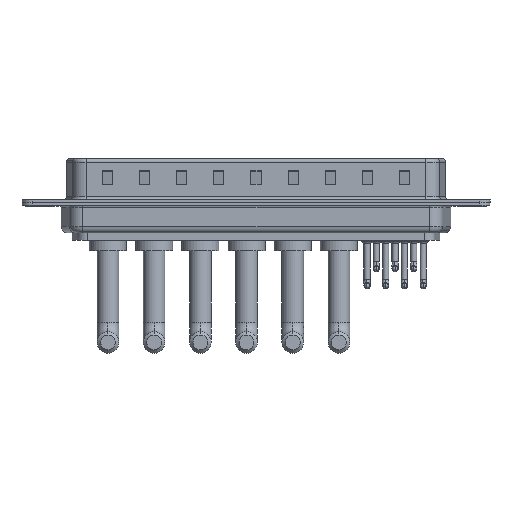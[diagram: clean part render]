
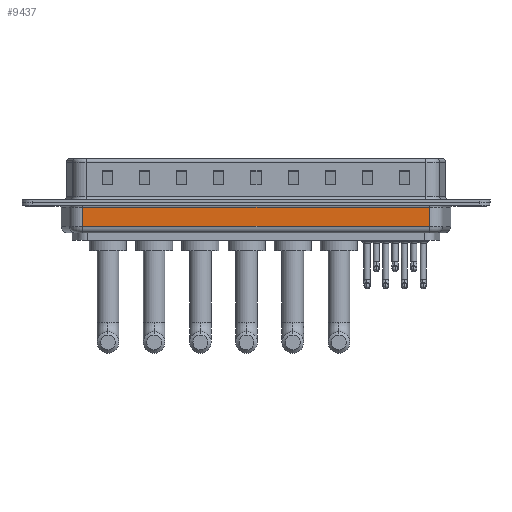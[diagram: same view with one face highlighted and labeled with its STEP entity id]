
A CAD part, front view. The second image highlights one B-rep face of the part: STEP entity #9437.
In plain terms, the highlighted planar face has unit normal (0, -1, 0).
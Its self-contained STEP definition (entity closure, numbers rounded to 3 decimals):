
#38 = VECTOR ( 'NONE', #15223, 1000. ) ;
#394 = CARTESIAN_POINT ( 'NONE',  ( 6.031, -5.35, -4.5 ) ) ;
#1238 = CARTESIAN_POINT ( 'NONE',  ( 57.469, -5.35, -3.5 ) ) ;
#1343 = VERTEX_POINT ( 'NONE', #16554 ) ;
#4052 = DIRECTION ( 'NONE',  ( -1., 0., 0. ) ) ;
#4387 = DIRECTION ( 'NONE',  ( 0., 0., 1. ) ) ;
#5097 = CARTESIAN_POINT ( 'NONE',  ( 6.031, -5.35, -0.65 ) ) ;
#5943 = VERTEX_POINT ( 'NONE', #10109 ) ;
#6286 = ORIENTED_EDGE ( 'NONE', *, *, #9462, .F. ) ;
#7620 = VERTEX_POINT ( 'NONE', #1238 ) ;
#8162 = ORIENTED_EDGE ( 'NONE', *, *, #16413, .T. ) ;
#8227 = CARTESIAN_POINT ( 'NONE',  ( 6.031, -5.35, -3.5 ) ) ;
#9286 = VECTOR ( 'NONE', #19094, 1000. ) ;
#9437 = ADVANCED_FACE ( 'NONE', ( #21397 ), #14633, .F. ) ;
#9462 = EDGE_CURVE ( 'NONE', #17589, #1343, #14866, .T. ) ;
#9883 = EDGE_CURVE ( 'NONE', #17589, #7620, #13262, .T. ) ;
#10109 = CARTESIAN_POINT ( 'NONE',  ( 57.469, -5.35, -0.65 ) ) ;
#10959 = CARTESIAN_POINT ( 'NONE',  ( 6.031, -5.35, -4.5 ) ) ;
#11719 = EDGE_CURVE ( 'NONE', #5943, #1343, #13826, .T. ) ;
#12854 = AXIS2_PLACEMENT_3D ( 'NONE', #10959, #17969, #4052 ) ;
#13262 = LINE ( 'NONE', #8227, #38 ) ;
#13292 = ORIENTED_EDGE ( 'NONE', *, *, #9883, .T. ) ;
#13826 = LINE ( 'NONE', #5097, #9286 ) ;
#14226 = EDGE_LOOP ( 'NONE', ( #6286, #13292, #8162, #15692 ) ) ;
#14633 = PLANE ( 'NONE',  #12854 ) ;
#14866 = LINE ( 'NONE', #394, #15432 ) ;
#15223 = DIRECTION ( 'NONE',  ( 1., 0., 0. ) ) ;
#15356 = DIRECTION ( 'NONE',  ( 0., 0., 1. ) ) ;
#15432 = VECTOR ( 'NONE', #4387, 1000. ) ;
#15692 = ORIENTED_EDGE ( 'NONE', *, *, #11719, .T. ) ;
#16329 = CARTESIAN_POINT ( 'NONE',  ( 6.031, -5.35, -3.5 ) ) ;
#16413 = EDGE_CURVE ( 'NONE', #7620, #5943, #16964, .T. ) ;
#16554 = CARTESIAN_POINT ( 'NONE',  ( 6.031, -5.35, -0.65 ) ) ;
#16964 = LINE ( 'NONE', #22242, #20409 ) ;
#17589 = VERTEX_POINT ( 'NONE', #16329 ) ;
#17969 = DIRECTION ( 'NONE',  ( 0., 1., 0. ) ) ;
#19094 = DIRECTION ( 'NONE',  ( -1., 0., 0. ) ) ;
#20409 = VECTOR ( 'NONE', #15356, 1000. ) ;
#21397 = FACE_OUTER_BOUND ( 'NONE', #14226, .T. ) ;
#22242 = CARTESIAN_POINT ( 'NONE',  ( 57.469, -5.35, -4.5 ) ) ;
